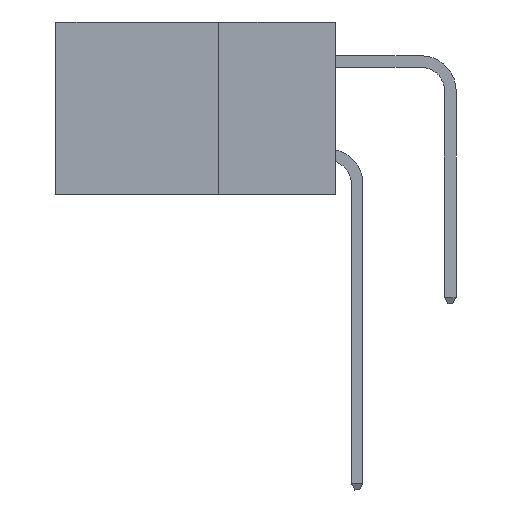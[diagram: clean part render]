
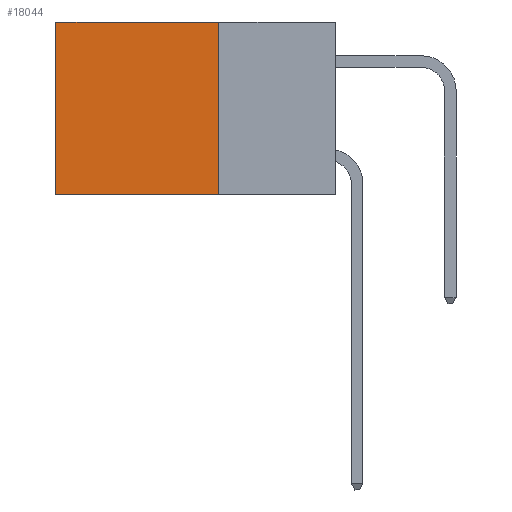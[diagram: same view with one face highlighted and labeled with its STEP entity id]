
A CAD part, left-side view. The second image highlights one B-rep face of the part: STEP entity #18044.
In plain terms, the highlighted planar face has unit normal (-1, 0, 0).
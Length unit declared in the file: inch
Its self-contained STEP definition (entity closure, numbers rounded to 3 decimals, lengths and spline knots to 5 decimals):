
#1574 = AXIS2_PLACEMENT_3D ( 'NONE', #13572, #18657, #13503 ) ;
#2153 = LINE ( 'NONE', #9352, #16433 ) ;
#2169 = VECTOR ( 'NONE', #19226, 39.37008 ) ;
#2546 = EDGE_CURVE ( 'NONE', #13855, #12949, #2684, .T. ) ;
#2684 = LINE ( 'NONE', #8149, #11745 ) ;
#2710 = EDGE_CURVE ( 'NONE', #12949, #13420, #7568, .T. ) ;
#2883 = DIRECTION ( 'NONE',  ( 0., 0., -1. ) ) ;
#4104 = CARTESIAN_POINT ( 'NONE',  ( 0.2875, 0.6, -0.37 ) ) ;
#4283 = DIRECTION ( 'NONE',  ( 0., 0., -1. ) ) ;
#5697 = ORIENTED_EDGE ( 'NONE', *, *, #2710, .F. ) ;
#7568 = LINE ( 'NONE', #10839, #2169 ) ;
#8149 = CARTESIAN_POINT ( 'NONE',  ( 0.2875, 0.25, 0. ) ) ;
#9210 = FACE_OUTER_BOUND ( 'NONE', #16710, .T. ) ;
#9352 = CARTESIAN_POINT ( 'NONE',  ( 0.2875, 0.6, 0. ) ) ;
#10839 = CARTESIAN_POINT ( 'NONE',  ( 0.2875, 0.25, -0.37 ) ) ;
#11130 = CARTESIAN_POINT ( 'NONE',  ( 0.2875, 0.25, 0. ) ) ;
#11202 = EDGE_CURVE ( 'NONE', #13855, #18043, #20516, .T. ) ;
#11745 = VECTOR ( 'NONE', #4283, 39.37008 ) ;
#11768 = CARTESIAN_POINT ( 'NONE',  ( 0.2875, 0.25, 0. ) ) ;
#11915 = ORIENTED_EDGE ( 'NONE', *, *, #20980, .T. ) ;
#12949 = VERTEX_POINT ( 'NONE', #20991 ) ;
#13420 = VERTEX_POINT ( 'NONE', #4104 ) ;
#13503 = DIRECTION ( 'NONE',  ( 0., 0., -1. ) ) ;
#13572 = CARTESIAN_POINT ( 'NONE',  ( 0.2875, 0.25, 0. ) ) ;
#13855 = VERTEX_POINT ( 'NONE', #11768 ) ;
#14497 = DIRECTION ( 'NONE',  ( 0., 1., 0. ) ) ;
#16095 = VECTOR ( 'NONE', #14497, 39.37008 ) ;
#16145 = ORIENTED_EDGE ( 'NONE', *, *, #2546, .F. ) ;
#16433 = VECTOR ( 'NONE', #2883, 39.37008 ) ;
#16710 = EDGE_LOOP ( 'NONE', ( #11915, #5697, #16145, #18303 ) ) ;
#18043 = VERTEX_POINT ( 'NONE', #19883 ) ;
#18044 = ADVANCED_FACE ( 'NONE', ( #9210 ), #20376, .F. ) ;
#18303 = ORIENTED_EDGE ( 'NONE', *, *, #11202, .T. ) ;
#18657 = DIRECTION ( 'NONE',  ( 1., 0., 0. ) ) ;
#19226 = DIRECTION ( 'NONE',  ( 0., 1., 0. ) ) ;
#19883 = CARTESIAN_POINT ( 'NONE',  ( 0.2875, 0.6, 0. ) ) ;
#20376 = PLANE ( 'NONE',  #1574 ) ;
#20516 = LINE ( 'NONE', #11130, #16095 ) ;
#20980 = EDGE_CURVE ( 'NONE', #18043, #13420, #2153, .T. ) ;
#20991 = CARTESIAN_POINT ( 'NONE',  ( 0.2875, 0.25, -0.37 ) ) ;
